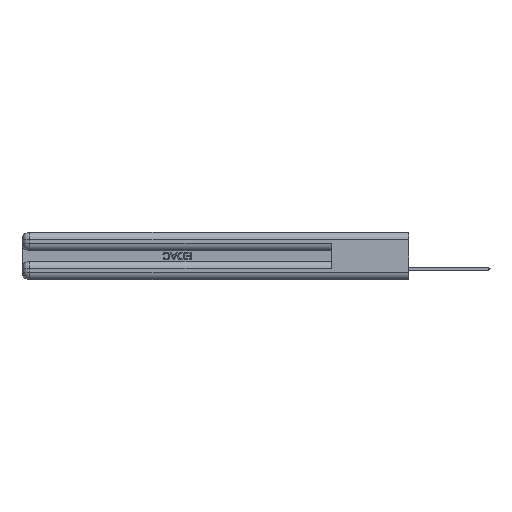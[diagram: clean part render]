
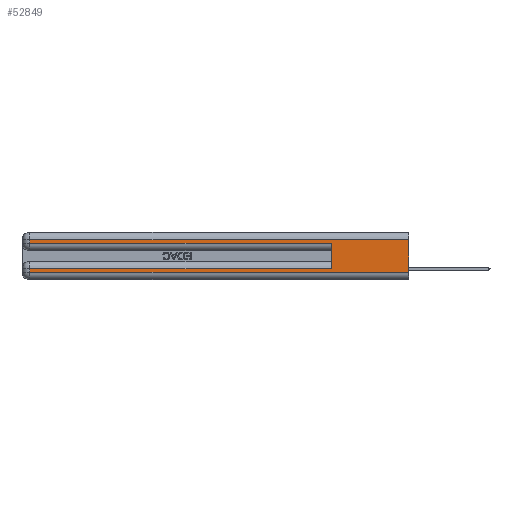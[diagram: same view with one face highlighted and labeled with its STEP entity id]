
A CAD part, left-side view. The second image highlights one B-rep face of the part: STEP entity #52849.
In plain terms, the highlighted planar face has unit normal (-1, 0, 0).
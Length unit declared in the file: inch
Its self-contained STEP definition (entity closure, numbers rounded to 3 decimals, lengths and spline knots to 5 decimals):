
#49 = LINE ( 'NONE', #19227, #13631 ) ;
#343 = VERTEX_POINT ( 'NONE', #25262 ) ;
#898 = EDGE_CURVE ( 'NONE', #21918, #32860, #19379, .T. ) ;
#2019 = VERTEX_POINT ( 'NONE', #41072 ) ;
#2464 = DIRECTION ( 'NONE',  ( 0., 0., -1. ) ) ;
#3039 = CARTESIAN_POINT ( 'NONE',  ( 0., 0., 0.06 ) ) ;
#4373 = CARTESIAN_POINT ( 'NONE',  ( 0., 2.94, 0.37 ) ) ;
#5183 = EDGE_LOOP ( 'NONE', ( #49417, #28554, #9717, #43243, #40339, #45183, #14080, #22673 ) ) ;
#5680 = CARTESIAN_POINT ( 'NONE',  ( 0., 0., 0.085 ) ) ;
#5863 = VERTEX_POINT ( 'NONE', #31596 ) ;
#6083 = CARTESIAN_POINT ( 'NONE',  ( 0., 0., 0.37 ) ) ;
#7245 = CARTESIAN_POINT ( 'NONE',  ( 0., 0., 0.31 ) ) ;
#9717 = ORIENTED_EDGE ( 'NONE', *, *, #39287, .T. ) ;
#10919 = VECTOR ( 'NONE', #29181, 39.37008 ) ;
#11224 = DIRECTION ( 'NONE',  ( 0., 1., 0. ) ) ;
#11490 = CARTESIAN_POINT ( 'NONE',  ( 0., 0., 0.285 ) ) ;
#12256 = DIRECTION ( 'NONE',  ( 0., -1., 0. ) ) ;
#12838 = VERTEX_POINT ( 'NONE', #50710 ) ;
#13631 = VECTOR ( 'NONE', #47941, 39.37008 ) ;
#13690 = EDGE_CURVE ( 'NONE', #17309, #343, #35374, .T. ) ;
#13776 = CARTESIAN_POINT ( 'NONE',  ( 0., 2.94, 0.085 ) ) ;
#13852 = EDGE_CURVE ( 'NONE', #5863, #343, #39304, .T. ) ;
#14080 = ORIENTED_EDGE ( 'NONE', *, *, #898, .T. ) ;
#14617 = PLANE ( 'NONE',  #17810 ) ;
#15141 = VECTOR ( 'NONE', #19652, 39.37008 ) ;
#17309 = VERTEX_POINT ( 'NONE', #34400 ) ;
#17810 = AXIS2_PLACEMENT_3D ( 'NONE', #6083, #31793, #2464 ) ;
#18725 = EDGE_CURVE ( 'NONE', #17309, #21918, #28921, .T. ) ;
#19122 = CARTESIAN_POINT ( 'NONE',  ( 0., 2.94, 0.31 ) ) ;
#19227 = CARTESIAN_POINT ( 'NONE',  ( 0., 0., 0.37 ) ) ;
#19379 = LINE ( 'NONE', #4373, #10919 ) ;
#19652 = DIRECTION ( 'NONE',  ( 0., -1., 0. ) ) ;
#20199 = VECTOR ( 'NONE', #12256, 39.37008 ) ;
#21860 = CARTESIAN_POINT ( 'NONE',  ( 0., 2.94, 0.06 ) ) ;
#21918 = VERTEX_POINT ( 'NONE', #13776 ) ;
#22673 = ORIENTED_EDGE ( 'NONE', *, *, #38953, .T. ) ;
#23879 = CARTESIAN_POINT ( 'NONE',  ( 0., 2.94, 0.37 ) ) ;
#24782 = EDGE_CURVE ( 'NONE', #12838, #36066, #50152, .T. ) ;
#24807 = CARTESIAN_POINT ( 'NONE',  ( 0., 0.6, 0.145 ) ) ;
#25262 = CARTESIAN_POINT ( 'NONE',  ( 0., 0.6, 0.285 ) ) ;
#27902 = VECTOR ( 'NONE', #11224, 39.37008 ) ;
#28554 = ORIENTED_EDGE ( 'NONE', *, *, #24782, .T. ) ;
#28921 = LINE ( 'NONE', #5680, #29537 ) ;
#29027 = DIRECTION ( 'NONE',  ( 0., 0., 1. ) ) ;
#29181 = DIRECTION ( 'NONE',  ( 0., 0., -1. ) ) ;
#29537 = VECTOR ( 'NONE', #39021, 39.37008 ) ;
#31596 = CARTESIAN_POINT ( 'NONE',  ( 0., 2.94, 0.285 ) ) ;
#31793 = DIRECTION ( 'NONE',  ( 1., 0., 0. ) ) ;
#32860 = VERTEX_POINT ( 'NONE', #21860 ) ;
#34400 = CARTESIAN_POINT ( 'NONE',  ( 0., 0.6, 0.085 ) ) ;
#35192 = LINE ( 'NONE', #3039, #20199 ) ;
#35374 = LINE ( 'NONE', #24807, #49186 ) ;
#36066 = VERTEX_POINT ( 'NONE', #19122 ) ;
#36526 = VECTOR ( 'NONE', #44745, 39.37008 ) ;
#38953 = EDGE_CURVE ( 'NONE', #32860, #2019, #35192, .T. ) ;
#39021 = DIRECTION ( 'NONE',  ( 0., 1., 0. ) ) ;
#39287 = EDGE_CURVE ( 'NONE', #36066, #5863, #52910, .T. ) ;
#39304 = LINE ( 'NONE', #11490, #15141 ) ;
#40339 = ORIENTED_EDGE ( 'NONE', *, *, #13690, .F. ) ;
#41072 = CARTESIAN_POINT ( 'NONE',  ( 0., 0., 0.06 ) ) ;
#43243 = ORIENTED_EDGE ( 'NONE', *, *, #13852, .T. ) ;
#44745 = DIRECTION ( 'NONE',  ( 0., 0., -1. ) ) ;
#45183 = ORIENTED_EDGE ( 'NONE', *, *, #18725, .T. ) ;
#47941 = DIRECTION ( 'NONE',  ( 0., 0., -1. ) ) ;
#48475 = EDGE_CURVE ( 'NONE', #12838, #2019, #49, .T. ) ;
#49186 = VECTOR ( 'NONE', #29027, 39.37008 ) ;
#49417 = ORIENTED_EDGE ( 'NONE', *, *, #48475, .F. ) ;
#50152 = LINE ( 'NONE', #7245, #27902 ) ;
#50710 = CARTESIAN_POINT ( 'NONE',  ( 0., 0., 0.31 ) ) ;
#52849 = ADVANCED_FACE ( 'NONE', ( #53378 ), #14617, .F. ) ;
#52910 = LINE ( 'NONE', #23879, #36526 ) ;
#53378 = FACE_OUTER_BOUND ( 'NONE', #5183, .T. ) ;
